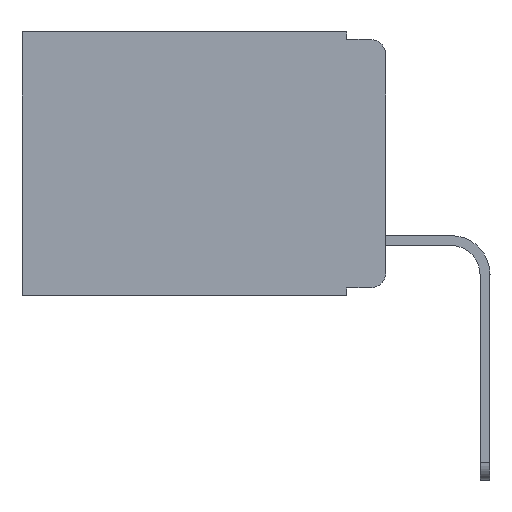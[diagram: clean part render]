
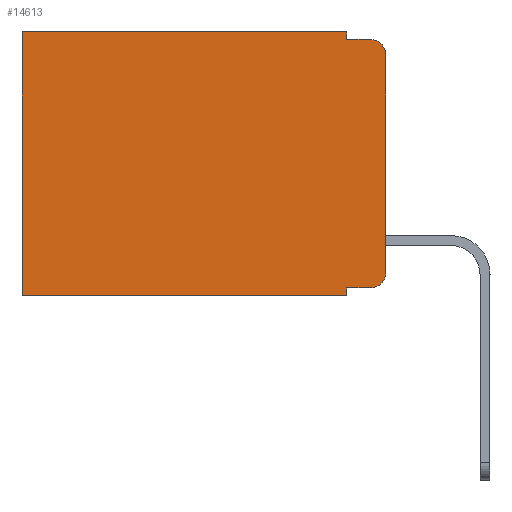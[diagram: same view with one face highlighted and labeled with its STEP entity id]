
A CAD part, left-side view. The second image highlights one B-rep face of the part: STEP entity #14613.
In plain terms, the highlighted planar face has unit normal (-1, 0, 0).
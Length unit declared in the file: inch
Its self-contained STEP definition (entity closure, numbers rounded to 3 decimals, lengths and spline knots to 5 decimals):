
#240 = EDGE_CURVE ( 'NONE', #252, #14872, #6958, .T. ) ;
#246 = ORIENTED_EDGE ( 'NONE', *, *, #240, .T. ) ;
#252 = VERTEX_POINT ( 'NONE', #2918 ) ;
#479 = DIRECTION ( 'NONE',  ( -1., 0., 0. ) ) ;
#585 = CARTESIAN_POINT ( 'NONE',  ( 0.298, 0.473, 0. ) ) ;
#652 = DIRECTION ( 'NONE',  ( 0., 0., -1. ) ) ;
#791 = CARTESIAN_POINT ( 'NONE',  ( 0.298, 0.051, -0.01 ) ) ;
#1142 = VECTOR ( 'NONE', #10910, 39.37008 ) ;
#1409 = EDGE_CURVE ( 'NONE', #5205, #14872, #12391, .T. ) ;
#1605 = DIRECTION ( 'NONE',  ( 0., 0., -1. ) ) ;
#1618 = LINE ( 'NONE', #4586, #2974 ) ;
#1904 = ORIENTED_EDGE ( 'NONE', *, *, #10897, .F. ) ;
#2297 = ORIENTED_EDGE ( 'NONE', *, *, #3481, .T. ) ;
#2350 = VERTEX_POINT ( 'NONE', #2614 ) ;
#2389 = LINE ( 'NONE', #4909, #10928 ) ;
#2614 = CARTESIAN_POINT ( 'NONE',  ( 0.298, 0.02, -0.01 ) ) ;
#2918 = CARTESIAN_POINT ( 'NONE',  ( 0.298, 0.02, -0.333 ) ) ;
#2974 = VECTOR ( 'NONE', #11795, 39.37008 ) ;
#2994 = VERTEX_POINT ( 'NONE', #13577 ) ;
#3259 = EDGE_CURVE ( 'NONE', #2994, #252, #11178, .T. ) ;
#3427 = VECTOR ( 'NONE', #7978, 39.37008 ) ;
#3481 = EDGE_CURVE ( 'NONE', #7008, #10096, #5842, .T. ) ;
#4059 = DIRECTION ( 'NONE',  ( 0., 0., -1. ) ) ;
#4110 = LINE ( 'NONE', #7762, #15133 ) ;
#4210 = CARTESIAN_POINT ( 'NONE',  ( 0.298, 0.473, -0.343 ) ) ;
#4333 = DIRECTION ( 'NONE',  ( -1., 0., 0. ) ) ;
#4586 = CARTESIAN_POINT ( 'NONE',  ( 0.298, 0.051, 0. ) ) ;
#4784 = VECTOR ( 'NONE', #9923, 39.37008 ) ;
#4797 = DIRECTION ( 'NONE',  ( 0., 1., 0. ) ) ;
#4879 = EDGE_CURVE ( 'NONE', #12890, #2350, #14456, .T. ) ;
#4909 = CARTESIAN_POINT ( 'NONE',  ( 0.298, 0., -0.343 ) ) ;
#5052 = EDGE_CURVE ( 'NONE', #5205, #2350, #12136, .T. ) ;
#5205 = VERTEX_POINT ( 'NONE', #9926 ) ;
#5542 = FACE_OUTER_BOUND ( 'NONE', #10092, .T. ) ;
#5722 = DIRECTION ( 'NONE',  ( 0., -1., 0. ) ) ;
#5842 = LINE ( 'NONE', #8948, #12985 ) ;
#6211 = AXIS2_PLACEMENT_3D ( 'NONE', #14049, #479, #4059 ) ;
#6267 = ORIENTED_EDGE ( 'NONE', *, *, #13954, .T. ) ;
#6428 = ORIENTED_EDGE ( 'NONE', *, *, #1409, .F. ) ;
#6935 = ORIENTED_EDGE ( 'NONE', *, *, #5052, .T. ) ;
#6958 = CIRCLE ( 'NONE', #6211, 0.02 ) ;
#7008 = VERTEX_POINT ( 'NONE', #585 ) ;
#7174 = ORIENTED_EDGE ( 'NONE', *, *, #3259, .T. ) ;
#7762 = CARTESIAN_POINT ( 'NONE',  ( 0.298, 0.051, 0. ) ) ;
#7833 = AXIS2_PLACEMENT_3D ( 'NONE', #9217, #4333, #652 ) ;
#7918 = VECTOR ( 'NONE', #5722, 39.37008 ) ;
#7978 = DIRECTION ( 'NONE',  ( 0., 1., 0. ) ) ;
#8104 = ORIENTED_EDGE ( 'NONE', *, *, #8155, .F. ) ;
#8155 = EDGE_CURVE ( 'NONE', #13078, #12890, #1618, .T. ) ;
#8235 = DIRECTION ( 'NONE',  ( 0., 0., -1. ) ) ;
#8441 = CARTESIAN_POINT ( 'NONE',  ( 0.298, 0., 0. ) ) ;
#8518 = AXIS2_PLACEMENT_3D ( 'NONE', #15278, #10792, #8235 ) ;
#8948 = CARTESIAN_POINT ( 'NONE',  ( 0.298, 0.473, 0. ) ) ;
#9217 = CARTESIAN_POINT ( 'NONE',  ( 0.298, 0.02, -0.03 ) ) ;
#9778 = CARTESIAN_POINT ( 'NONE',  ( 0.298, 0., -0.313 ) ) ;
#9923 = DIRECTION ( 'NONE',  ( 0., -1., 0. ) ) ;
#9926 = CARTESIAN_POINT ( 'NONE',  ( 0.298, 0., -0.03 ) ) ;
#10075 = CARTESIAN_POINT ( 'NONE',  ( 0.298, 0.051, -0.333 ) ) ;
#10092 = EDGE_LOOP ( 'NONE', ( #6428, #6935, #14308, #8104, #6267, #2297, #12004, #1904, #7174, #246 ) ) ;
#10096 = VERTEX_POINT ( 'NONE', #4210 ) ;
#10451 = CARTESIAN_POINT ( 'NONE',  ( 0.298, 0.051, -0.01 ) ) ;
#10497 = DIRECTION ( 'NONE',  ( 0., 0., -1. ) ) ;
#10792 = DIRECTION ( 'NONE',  ( 1., 0., 0. ) ) ;
#10897 = EDGE_CURVE ( 'NONE', #2994, #14487, #4110, .T. ) ;
#10910 = DIRECTION ( 'NONE',  ( 0., 0., -1. ) ) ;
#10928 = VECTOR ( 'NONE', #4797, 39.37008 ) ;
#11178 = LINE ( 'NONE', #10075, #4784 ) ;
#11795 = DIRECTION ( 'NONE',  ( 0., 0., -1. ) ) ;
#11826 = PLANE ( 'NONE',  #8518 ) ;
#12004 = ORIENTED_EDGE ( 'NONE', *, *, #15936, .F. ) ;
#12136 = CIRCLE ( 'NONE', #7833, 0.02 ) ;
#12349 = LINE ( 'NONE', #12816, #3427 ) ;
#12391 = LINE ( 'NONE', #8441, #1142 ) ;
#12816 = CARTESIAN_POINT ( 'NONE',  ( 0.298, 0., 0. ) ) ;
#12890 = VERTEX_POINT ( 'NONE', #10451 ) ;
#12985 = VECTOR ( 'NONE', #10497, 39.37008 ) ;
#13078 = VERTEX_POINT ( 'NONE', #15963 ) ;
#13577 = CARTESIAN_POINT ( 'NONE',  ( 0.298, 0.051, -0.333 ) ) ;
#13954 = EDGE_CURVE ( 'NONE', #13078, #7008, #12349, .T. ) ;
#14049 = CARTESIAN_POINT ( 'NONE',  ( 0.298, 0.02, -0.313 ) ) ;
#14308 = ORIENTED_EDGE ( 'NONE', *, *, #4879, .F. ) ;
#14456 = LINE ( 'NONE', #791, #7918 ) ;
#14487 = VERTEX_POINT ( 'NONE', #15167 ) ;
#14613 = ADVANCED_FACE ( 'NONE', ( #5542 ), #11826, .F. ) ;
#14872 = VERTEX_POINT ( 'NONE', #9778 ) ;
#15133 = VECTOR ( 'NONE', #1605, 39.37008 ) ;
#15167 = CARTESIAN_POINT ( 'NONE',  ( 0.298, 0.051, -0.343 ) ) ;
#15278 = CARTESIAN_POINT ( 'NONE',  ( 0.298, 0., 0. ) ) ;
#15936 = EDGE_CURVE ( 'NONE', #14487, #10096, #2389, .T. ) ;
#15963 = CARTESIAN_POINT ( 'NONE',  ( 0.298, 0.051, 0. ) ) ;
